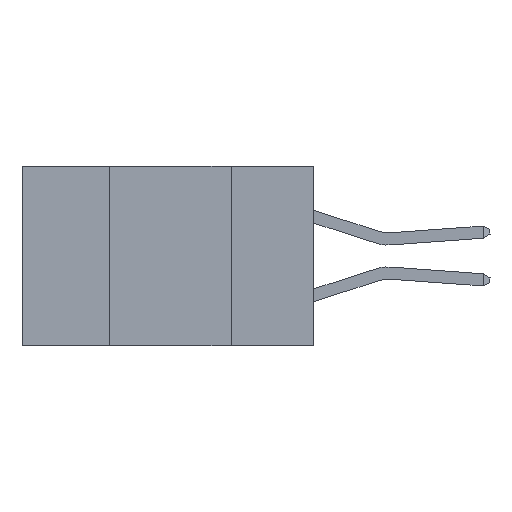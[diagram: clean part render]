
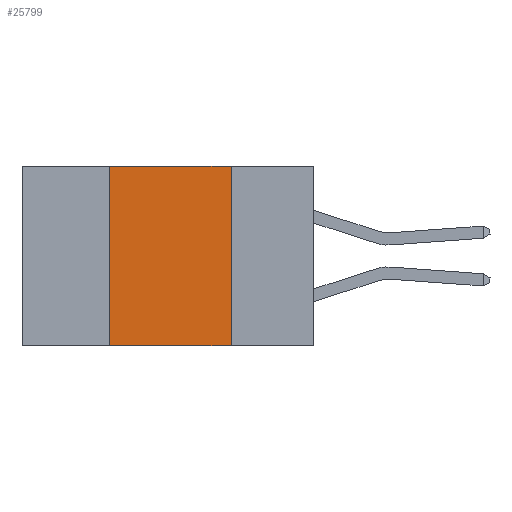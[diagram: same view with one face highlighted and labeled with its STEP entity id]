
A CAD part, left-side view. The second image highlights one B-rep face of the part: STEP entity #25799.
In plain terms, the highlighted planar face has unit normal (-1, 0, 0).
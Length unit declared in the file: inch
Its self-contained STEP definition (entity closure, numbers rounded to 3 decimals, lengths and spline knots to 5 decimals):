
#919 = CARTESIAN_POINT ( 'NONE',  ( 0., 0.6, -0.37 ) ) ;
#1788 = ORIENTED_EDGE ( 'NONE', *, *, #4760, .F. ) ;
#4760 = EDGE_CURVE ( 'NONE', #25076, #4861, #17149, .T. ) ;
#4861 = VERTEX_POINT ( 'NONE', #19808 ) ;
#5664 = CARTESIAN_POINT ( 'NONE',  ( 0., 0.6, 0. ) ) ;
#5746 = LINE ( 'NONE', #14145, #24179 ) ;
#5890 = DIRECTION ( 'NONE',  ( 0., -1., 0. ) ) ;
#6746 = VECTOR ( 'NONE', #29331, 39.37008 ) ;
#7825 = CARTESIAN_POINT ( 'NONE',  ( 0., 0.17, 0. ) ) ;
#9836 = CARTESIAN_POINT ( 'NONE',  ( 0., 0.42, 0. ) ) ;
#9966 = VECTOR ( 'NONE', #19498, 39.37008 ) ;
#10160 = ORIENTED_EDGE ( 'NONE', *, *, #19535, .F. ) ;
#10633 = CARTESIAN_POINT ( 'NONE',  ( 0., 0.17, -0.37 ) ) ;
#12509 = VERTEX_POINT ( 'NONE', #22194 ) ;
#13188 = LINE ( 'NONE', #7825, #6746 ) ;
#14145 = CARTESIAN_POINT ( 'NONE',  ( 0., 0.6, 0. ) ) ;
#15430 = DIRECTION ( 'NONE',  ( 0., 0., -1. ) ) ;
#16411 = AXIS2_PLACEMENT_3D ( 'NONE', #5664, #29616, #15430 ) ;
#16953 = DIRECTION ( 'NONE',  ( 0., -1., 0. ) ) ;
#17149 = LINE ( 'NONE', #9836, #9966 ) ;
#17378 = LINE ( 'NONE', #919, #29964 ) ;
#17621 = EDGE_LOOP ( 'NONE', ( #23558, #10160, #1788, #24557 ) ) ;
#19498 = DIRECTION ( 'NONE',  ( 0., 0., 1. ) ) ;
#19535 = EDGE_CURVE ( 'NONE', #4861, #12509, #5746, .T. ) ;
#19808 = CARTESIAN_POINT ( 'NONE',  ( 0., 0.42, 0. ) ) ;
#21927 = EDGE_CURVE ( 'NONE', #12509, #24603, #13188, .T. ) ;
#22135 = CARTESIAN_POINT ( 'NONE',  ( 0., 0.42, -0.37 ) ) ;
#22194 = CARTESIAN_POINT ( 'NONE',  ( 0., 0.17, 0. ) ) ;
#22514 = PLANE ( 'NONE',  #16411 ) ;
#23558 = ORIENTED_EDGE ( 'NONE', *, *, #21927, .F. ) ;
#24179 = VECTOR ( 'NONE', #16953, 39.37008 ) ;
#24557 = ORIENTED_EDGE ( 'NONE', *, *, #26918, .T. ) ;
#24603 = VERTEX_POINT ( 'NONE', #10633 ) ;
#25076 = VERTEX_POINT ( 'NONE', #22135 ) ;
#25665 = FACE_OUTER_BOUND ( 'NONE', #17621, .T. ) ;
#25799 = ADVANCED_FACE ( 'NONE', ( #25665 ), #22514, .F. ) ;
#26918 = EDGE_CURVE ( 'NONE', #25076, #24603, #17378, .T. ) ;
#29331 = DIRECTION ( 'NONE',  ( 0., 0., -1. ) ) ;
#29616 = DIRECTION ( 'NONE',  ( 1., 0., 0. ) ) ;
#29964 = VECTOR ( 'NONE', #5890, 39.37008 ) ;
